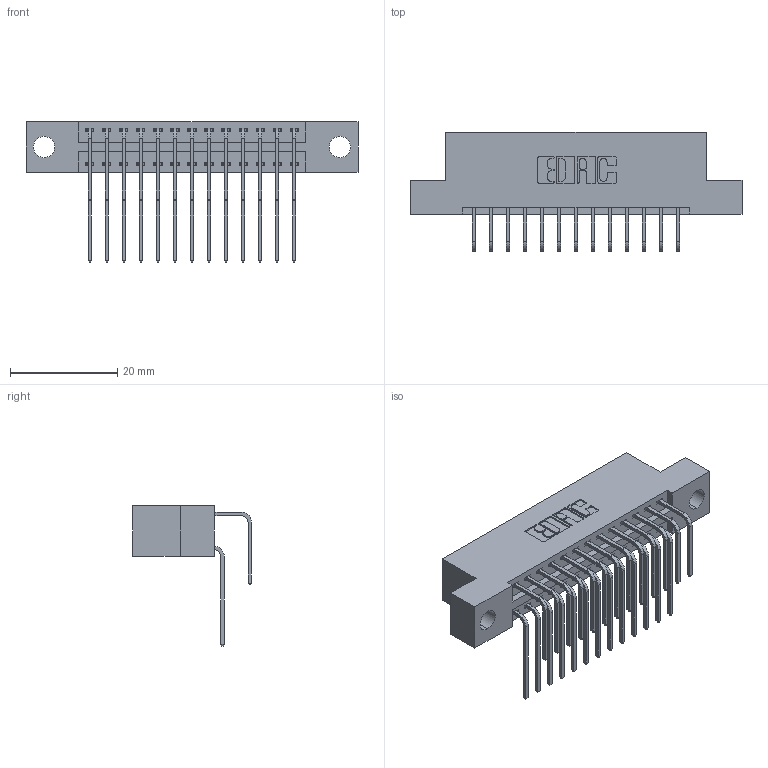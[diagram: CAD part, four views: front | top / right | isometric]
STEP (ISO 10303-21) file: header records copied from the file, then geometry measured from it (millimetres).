
FILE_DESCRIPTION (( 'STEP AP203' ), '1' );
FILE_NAME ('346-026-558-204.STEP', '2022-05-19T02:42:03', ( '' ), ( '' ), 'SwSTEP 2.0', 'SolidWorks 2020', '' );
FILE_SCHEMA (( 'CONFIG_CONTROL_DESIGN' ));
Length unit declared in the file: inch
Products named in the file (4): 345-292-001_558 559 Tail - 1; 346 Part_Flush Mounting Lugs - 0.156 Dia-TH; 345-292-001_558 Tail - 2; 346-026-558-204
Assembly tree (27 placements, depth 2):
  346-026-558-204
    346 Part_Flush Mounting Lugs - 0.156 Dia-TH
    345-292-001_558 559 Tail - 1  x13
    345-292-001_558 Tail - 2  x13
Bounding box: 61.85 x 22.16 x 26.16 mm (x, y, z)
Volume: 5849.8 mm3; surface area: 8152.6 mm2
Topology: 27 solids, 27 shells, 1540 faces, 4551 edges, 2998 vertices
Faces by surface type: plane 1052, cylinder 488
Entity records: 14591 total; most frequent: CARTESIAN_POINT 2501, ORIENTED_EDGE 2382, DIRECTION 2227, EDGE_CURVE 1191, VECTOR 967, LINE 967, VERTEX_POINT 790, AXIS2_PLACEMENT_3D 630
